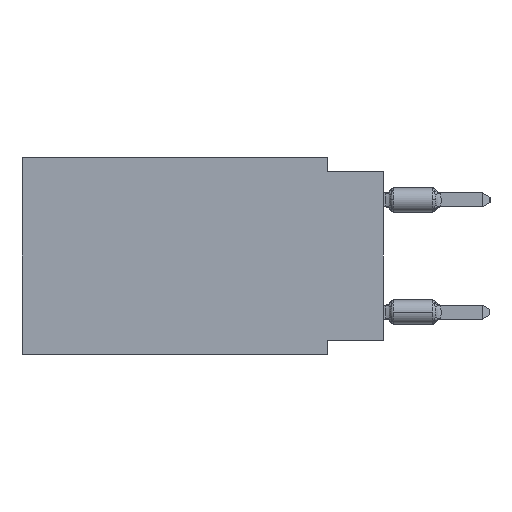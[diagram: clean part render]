
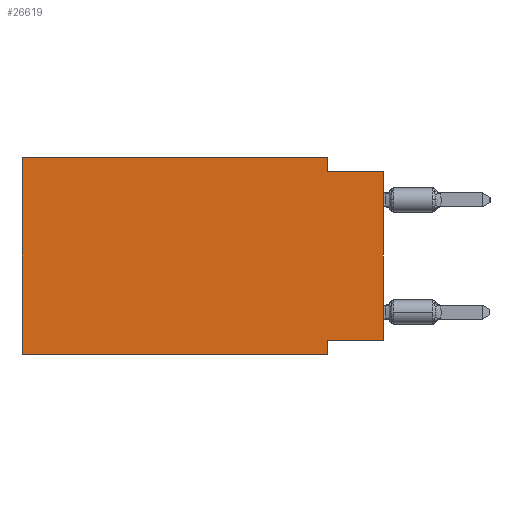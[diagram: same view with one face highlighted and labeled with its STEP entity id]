
A CAD part, left-side view. The second image highlights one B-rep face of the part: STEP entity #26619.
In plain terms, the highlighted planar face has unit normal (-1, 0, 0).
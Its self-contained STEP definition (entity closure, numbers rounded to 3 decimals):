
#2051 = ORIENTED_EDGE ( 'NONE', *, *, #28183, .F. ) ;
#2202 = EDGE_CURVE ( 'NONE', #5024, #19867, #7754, .T. ) ;
#2275 = VECTOR ( 'NONE', #13459, 1000. ) ;
#3039 = CARTESIAN_POINT ( 'NONE',  ( 0., 16.383, 0. ) ) ;
#3323 = DIRECTION ( 'NONE',  ( 0., 0., -1. ) ) ;
#3414 = CARTESIAN_POINT ( 'NONE',  ( 0., 16.383, -8.89 ) ) ;
#3616 = DIRECTION ( 'NONE',  ( 0., 1., 0. ) ) ;
#3683 = CARTESIAN_POINT ( 'NONE',  ( 0., 16.383, 0. ) ) ;
#3725 = AXIS2_PLACEMENT_3D ( 'NONE', #3039, #21109, #18738 ) ;
#4306 = VECTOR ( 'NONE', #3616, 1000. ) ;
#5024 = VERTEX_POINT ( 'NONE', #21440 ) ;
#5758 = DIRECTION ( 'NONE',  ( 0., -1., 0. ) ) ;
#6401 = DIRECTION ( 'NONE',  ( 0., 0., 1. ) ) ;
#6846 = EDGE_CURVE ( 'NONE', #19867, #8551, #21984, .T. ) ;
#7321 = ORIENTED_EDGE ( 'NONE', *, *, #2202, .F. ) ;
#7411 = EDGE_CURVE ( 'NONE', #25822, #28597, #22246, .T. ) ;
#7570 = DIRECTION ( 'NONE',  ( 0., -1., 0. ) ) ;
#7732 = VECTOR ( 'NONE', #3323, 1000. ) ;
#7754 = LINE ( 'NONE', #25816, #7732 ) ;
#8169 = LINE ( 'NONE', #23993, #21681 ) ;
#8215 = CARTESIAN_POINT ( 'NONE',  ( 0., 0., -8.255 ) ) ;
#8551 = VERTEX_POINT ( 'NONE', #16645 ) ;
#8591 = VERTEX_POINT ( 'NONE', #28036 ) ;
#8982 = ORIENTED_EDGE ( 'NONE', *, *, #7411, .F. ) ;
#9859 = ORIENTED_EDGE ( 'NONE', *, *, #14262, .F. ) ;
#10299 = CARTESIAN_POINT ( 'NONE',  ( 0., 0., -0.635 ) ) ;
#10993 = CARTESIAN_POINT ( 'NONE',  ( 0., 2.54, -8.89 ) ) ;
#11053 = EDGE_CURVE ( 'NONE', #8591, #8551, #13384, .T. ) ;
#11920 = CARTESIAN_POINT ( 'NONE',  ( 0., 2.54, -8.255 ) ) ;
#13384 = LINE ( 'NONE', #24755, #26856 ) ;
#13459 = DIRECTION ( 'NONE',  ( 0., 0., -1. ) ) ;
#13610 = EDGE_LOOP ( 'NONE', ( #26001, #20067, #7321, #9859, #8982, #22739, #2051, #27001 ) ) ;
#14169 = VECTOR ( 'NONE', #5758, 1000. ) ;
#14262 = EDGE_CURVE ( 'NONE', #28597, #5024, #26636, .T. ) ;
#14903 = DIRECTION ( 'NONE',  ( 0., -1., 0. ) ) ;
#15823 = VECTOR ( 'NONE', #14903, 1000. ) ;
#16391 = FACE_OUTER_BOUND ( 'NONE', #13610, .T. ) ;
#16645 = CARTESIAN_POINT ( 'NONE',  ( 0., 0., -0.635 ) ) ;
#17033 = VERTEX_POINT ( 'NONE', #11920 ) ;
#18738 = DIRECTION ( 'NONE',  ( 0., 0., -1. ) ) ;
#18889 = PLANE ( 'NONE',  #3725 ) ;
#19867 = VERTEX_POINT ( 'NONE', #24572 ) ;
#20067 = ORIENTED_EDGE ( 'NONE', *, *, #6846, .F. ) ;
#20169 = CARTESIAN_POINT ( 'NONE',  ( 0., 16.383, 0. ) ) ;
#21109 = DIRECTION ( 'NONE',  ( 1., 0., 0. ) ) ;
#21346 = VERTEX_POINT ( 'NONE', #10993 ) ;
#21440 = CARTESIAN_POINT ( 'NONE',  ( 0., 2.54, 0. ) ) ;
#21681 = VECTOR ( 'NONE', #7570, 1000. ) ;
#21978 = VECTOR ( 'NONE', #22681, 1000. ) ;
#21984 = LINE ( 'NONE', #10299, #15823 ) ;
#22246 = LINE ( 'NONE', #20169, #21978 ) ;
#22681 = DIRECTION ( 'NONE',  ( 0., 0., 1. ) ) ;
#22739 = ORIENTED_EDGE ( 'NONE', *, *, #28711, .T. ) ;
#23993 = CARTESIAN_POINT ( 'NONE',  ( 0., 16.383, -8.89 ) ) ;
#24199 = LINE ( 'NONE', #8215, #4306 ) ;
#24572 = CARTESIAN_POINT ( 'NONE',  ( 0., 2.54, -0.635 ) ) ;
#24755 = CARTESIAN_POINT ( 'NONE',  ( 0., 0., 0. ) ) ;
#24980 = LINE ( 'NONE', #27063, #2275 ) ;
#25816 = CARTESIAN_POINT ( 'NONE',  ( 0., 2.54, 0. ) ) ;
#25822 = VERTEX_POINT ( 'NONE', #3414 ) ;
#26001 = ORIENTED_EDGE ( 'NONE', *, *, #11053, .T. ) ;
#26619 = ADVANCED_FACE ( 'NONE', ( #16391 ), #18889, .F. ) ;
#26636 = LINE ( 'NONE', #3683, #14169 ) ;
#26856 = VECTOR ( 'NONE', #6401, 1000. ) ;
#27001 = ORIENTED_EDGE ( 'NONE', *, *, #27820, .F. ) ;
#27063 = CARTESIAN_POINT ( 'NONE',  ( 0., 2.54, -8.89 ) ) ;
#27717 = CARTESIAN_POINT ( 'NONE',  ( 0., 16.383, 0. ) ) ;
#27820 = EDGE_CURVE ( 'NONE', #8591, #17033, #24199, .T. ) ;
#28036 = CARTESIAN_POINT ( 'NONE',  ( 0., 0., -8.255 ) ) ;
#28183 = EDGE_CURVE ( 'NONE', #17033, #21346, #24980, .T. ) ;
#28597 = VERTEX_POINT ( 'NONE', #27717 ) ;
#28711 = EDGE_CURVE ( 'NONE', #25822, #21346, #8169, .T. ) ;
